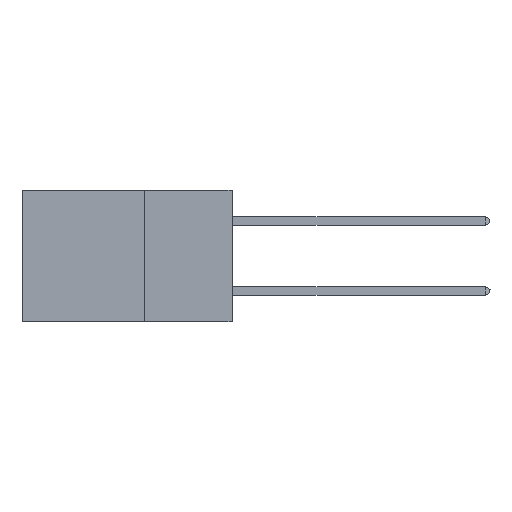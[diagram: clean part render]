
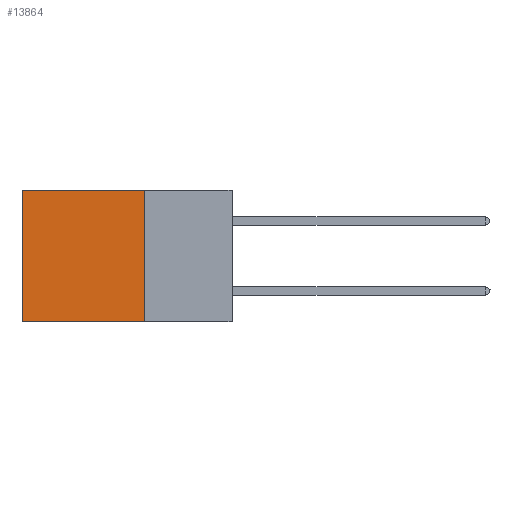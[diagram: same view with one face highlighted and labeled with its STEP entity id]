
A CAD part, left-side view. The second image highlights one B-rep face of the part: STEP entity #13864.
In plain terms, the highlighted planar face has unit normal (-1, 0, 0).
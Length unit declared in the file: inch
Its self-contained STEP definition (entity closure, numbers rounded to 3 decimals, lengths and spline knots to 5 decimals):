
#470 = CARTESIAN_POINT ( 'NONE',  ( 0.2875, 0.25, -0.375 ) ) ;
#836 = LINE ( 'NONE', #3444, #13085 ) ;
#1042 = FACE_OUTER_BOUND ( 'NONE', #8408, .T. ) ;
#1063 = ORIENTED_EDGE ( 'NONE', *, *, #9170, .T. ) ;
#1561 = EDGE_CURVE ( 'NONE', #13087, #14509, #836, .T. ) ;
#1807 = CARTESIAN_POINT ( 'NONE',  ( 0.2875, 0.25, -0.375 ) ) ;
#2171 = CARTESIAN_POINT ( 'NONE',  ( 0.2875, 0.25, 0. ) ) ;
#3444 = CARTESIAN_POINT ( 'NONE',  ( 0.2875, 0.6, -0.375 ) ) ;
#3818 = VECTOR ( 'NONE', #12691, 39.37008 ) ;
#4499 = LINE ( 'NONE', #1807, #13703 ) ;
#4637 = CARTESIAN_POINT ( 'NONE',  ( 0.2875, 0.25, -0.375 ) ) ;
#5361 = ORIENTED_EDGE ( 'NONE', *, *, #14397, .F. ) ;
#5805 = DIRECTION ( 'NONE',  ( 0., 0., -1. ) ) ;
#5866 = VERTEX_POINT ( 'NONE', #470 ) ;
#6616 = PLANE ( 'NONE',  #12244 ) ;
#8095 = EDGE_CURVE ( 'NONE', #5866, #14509, #14569, .T. ) ;
#8408 = EDGE_LOOP ( 'NONE', ( #15815, #15432, #5361, #1063 ) ) ;
#9058 = DIRECTION ( 'NONE',  ( 1., 0., 0. ) ) ;
#9170 = EDGE_CURVE ( 'NONE', #14074, #13087, #12011, .T. ) ;
#10091 = CARTESIAN_POINT ( 'NONE',  ( 0.2875, 0.6, 0. ) ) ;
#10815 = CARTESIAN_POINT ( 'NONE',  ( 0.2875, 0.25, 0. ) ) ;
#11243 = DIRECTION ( 'NONE',  ( 0., 1., 0. ) ) ;
#11687 = DIRECTION ( 'NONE',  ( 0., 0., -1. ) ) ;
#12011 = LINE ( 'NONE', #2171, #3818 ) ;
#12244 = AXIS2_PLACEMENT_3D ( 'NONE', #15785, #9058, #11687 ) ;
#12691 = DIRECTION ( 'NONE',  ( 0., 1., 0. ) ) ;
#13085 = VECTOR ( 'NONE', #13889, 39.37008 ) ;
#13087 = VERTEX_POINT ( 'NONE', #10091 ) ;
#13571 = VECTOR ( 'NONE', #11243, 39.37008 ) ;
#13703 = VECTOR ( 'NONE', #5805, 39.37008 ) ;
#13864 = ADVANCED_FACE ( 'NONE', ( #1042 ), #6616, .F. ) ;
#13889 = DIRECTION ( 'NONE',  ( 0., 0., -1. ) ) ;
#14074 = VERTEX_POINT ( 'NONE', #10815 ) ;
#14397 = EDGE_CURVE ( 'NONE', #14074, #5866, #4499, .T. ) ;
#14509 = VERTEX_POINT ( 'NONE', #16433 ) ;
#14569 = LINE ( 'NONE', #4637, #13571 ) ;
#15432 = ORIENTED_EDGE ( 'NONE', *, *, #8095, .F. ) ;
#15785 = CARTESIAN_POINT ( 'NONE',  ( 0.2875, 0.25, -0.375 ) ) ;
#15815 = ORIENTED_EDGE ( 'NONE', *, *, #1561, .T. ) ;
#16433 = CARTESIAN_POINT ( 'NONE',  ( 0.2875, 0.6, -0.375 ) ) ;
